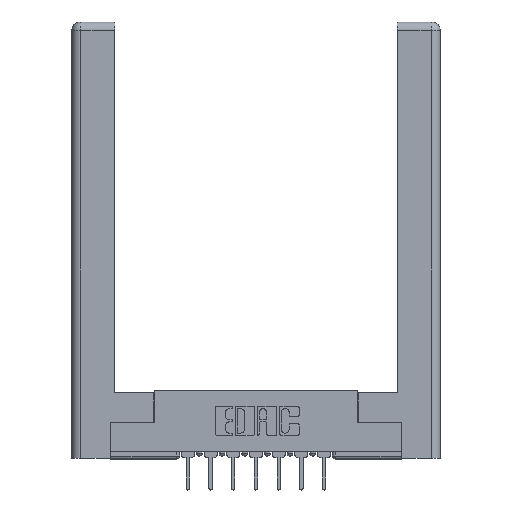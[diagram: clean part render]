
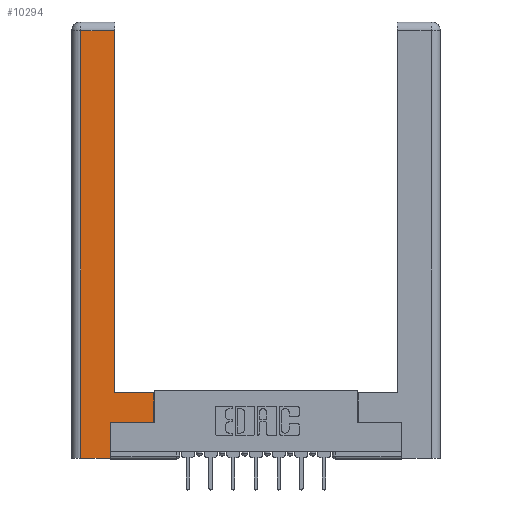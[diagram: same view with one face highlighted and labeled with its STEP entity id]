
A CAD part, top view. The second image highlights one B-rep face of the part: STEP entity #10294.
In plain terms, the highlighted planar face has unit normal (0, 0, 1).
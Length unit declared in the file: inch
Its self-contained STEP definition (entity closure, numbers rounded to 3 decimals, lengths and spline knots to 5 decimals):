
#156 = LINE ( 'NONE', #13134, #2998 ) ;
#162 = LINE ( 'NONE', #10106, #2112 ) ;
#359 = ORIENTED_EDGE ( 'NONE', *, *, #8710, .T. ) ;
#449 = VECTOR ( 'NONE', #12280, 39.37008 ) ;
#1067 = CARTESIAN_POINT ( 'NONE',  ( 0.265, 0., 0. ) ) ;
#1276 = VECTOR ( 'NONE', #12469, 39.37008 ) ;
#1563 = ORIENTED_EDGE ( 'NONE', *, *, #12402, .T. ) ;
#1958 = ORIENTED_EDGE ( 'NONE', *, *, #6065, .T. ) ;
#2043 = LINE ( 'NONE', #2914, #12171 ) ;
#2112 = VECTOR ( 'NONE', #11327, 39.37008 ) ;
#2207 = EDGE_LOOP ( 'NONE', ( #8589, #6476, #9146, #359, #4126, #1563, #1958, #5641 ) ) ;
#2210 = VERTEX_POINT ( 'NONE', #4223 ) ;
#2227 = CARTESIAN_POINT ( 'NONE',  ( 0.565, 0.45, 0. ) ) ;
#2521 = VERTEX_POINT ( 'NONE', #8510 ) ;
#2914 = CARTESIAN_POINT ( 'NONE',  ( 0.295, 3., 0. ) ) ;
#2935 = LINE ( 'NONE', #11228, #5227 ) ;
#2998 = VECTOR ( 'NONE', #5265, 39.37008 ) ;
#3010 = EDGE_CURVE ( 'NONE', #4354, #4479, #7861, .T. ) ;
#3201 = VERTEX_POINT ( 'NONE', #2227 ) ;
#3489 = AXIS2_PLACEMENT_3D ( 'NONE', #7856, #7921, #9801 ) ;
#3567 = VECTOR ( 'NONE', #9810, 39.37008 ) ;
#3738 = VECTOR ( 'NONE', #6576, 39.37008 ) ;
#3871 = EDGE_CURVE ( 'NONE', #4994, #2210, #162, .T. ) ;
#4126 = ORIENTED_EDGE ( 'NONE', *, *, #3871, .T. ) ;
#4223 = CARTESIAN_POINT ( 'NONE',  ( 0.265, 0.245, 0. ) ) ;
#4354 = VERTEX_POINT ( 'NONE', #12360 ) ;
#4418 = VERTEX_POINT ( 'NONE', #12851 ) ;
#4479 = VERTEX_POINT ( 'NONE', #4727 ) ;
#4727 = CARTESIAN_POINT ( 'NONE',  ( 0.0615, 2.94, 0. ) ) ;
#4994 = VERTEX_POINT ( 'NONE', #1067 ) ;
#5227 = VECTOR ( 'NONE', #9195, 39.37008 ) ;
#5265 = DIRECTION ( 'NONE',  ( 0., -1., 0. ) ) ;
#5370 = EDGE_CURVE ( 'NONE', #4479, #4418, #156, .T. ) ;
#5641 = ORIENTED_EDGE ( 'NONE', *, *, #12621, .T. ) ;
#6065 = EDGE_CURVE ( 'NONE', #12147, #3201, #8407, .T. ) ;
#6476 = ORIENTED_EDGE ( 'NONE', *, *, #3010, .T. ) ;
#6576 = DIRECTION ( 'NONE',  ( 1., 0., 0. ) ) ;
#6844 = CARTESIAN_POINT ( 'NONE',  ( 0.565, 0.245, 0. ) ) ;
#7736 = LINE ( 'NONE', #10908, #3738 ) ;
#7856 = CARTESIAN_POINT ( 'NONE',  ( 0., 0., 0. ) ) ;
#7861 = LINE ( 'NONE', #11694, #3567 ) ;
#7921 = DIRECTION ( 'NONE',  ( 0., 0., -1. ) ) ;
#8407 = LINE ( 'NONE', #11367, #1276 ) ;
#8510 = CARTESIAN_POINT ( 'NONE',  ( 0.295, 0.45, 0. ) ) ;
#8589 = ORIENTED_EDGE ( 'NONE', *, *, #10858, .T. ) ;
#8710 = EDGE_CURVE ( 'NONE', #4418, #4994, #10221, .T. ) ;
#8788 = PLANE ( 'NONE',  #3489 ) ;
#9146 = ORIENTED_EDGE ( 'NONE', *, *, #5370, .T. ) ;
#9195 = DIRECTION ( 'NONE',  ( -1., 0., 0. ) ) ;
#9203 = CARTESIAN_POINT ( 'NONE',  ( 0.265, 0., 0. ) ) ;
#9729 = FACE_OUTER_BOUND ( 'NONE', #2207, .T. ) ;
#9801 = DIRECTION ( 'NONE',  ( -1., 0., 0. ) ) ;
#9810 = DIRECTION ( 'NONE',  ( -1., 0., 0. ) ) ;
#10106 = CARTESIAN_POINT ( 'NONE',  ( 0.265, 0.245, 0. ) ) ;
#10221 = LINE ( 'NONE', #9203, #449 ) ;
#10294 = ADVANCED_FACE ( 'NONE', ( #9729 ), #8788, .F. ) ;
#10858 = EDGE_CURVE ( 'NONE', #2521, #4354, #2043, .T. ) ;
#10908 = CARTESIAN_POINT ( 'NONE',  ( 0.565, 0.245, 0. ) ) ;
#11228 = CARTESIAN_POINT ( 'NONE',  ( 0.295, 0.45, 0. ) ) ;
#11327 = DIRECTION ( 'NONE',  ( 0., 1., 0. ) ) ;
#11367 = CARTESIAN_POINT ( 'NONE',  ( 0.565, 0.45, 0. ) ) ;
#11694 = CARTESIAN_POINT ( 'NONE',  ( 0.0615, 2.94, 0. ) ) ;
#12147 = VERTEX_POINT ( 'NONE', #6844 ) ;
#12171 = VECTOR ( 'NONE', #12254, 39.37008 ) ;
#12254 = DIRECTION ( 'NONE',  ( 0., 1., 0. ) ) ;
#12280 = DIRECTION ( 'NONE',  ( 1., 0., 0. ) ) ;
#12360 = CARTESIAN_POINT ( 'NONE',  ( 0.295, 2.94, 0. ) ) ;
#12402 = EDGE_CURVE ( 'NONE', #2210, #12147, #7736, .T. ) ;
#12469 = DIRECTION ( 'NONE',  ( 0., 1., 0. ) ) ;
#12621 = EDGE_CURVE ( 'NONE', #3201, #2521, #2935, .T. ) ;
#12851 = CARTESIAN_POINT ( 'NONE',  ( 0.0615, 0., 0. ) ) ;
#13134 = CARTESIAN_POINT ( 'NONE',  ( 0.0615, 0., 0. ) ) ;
